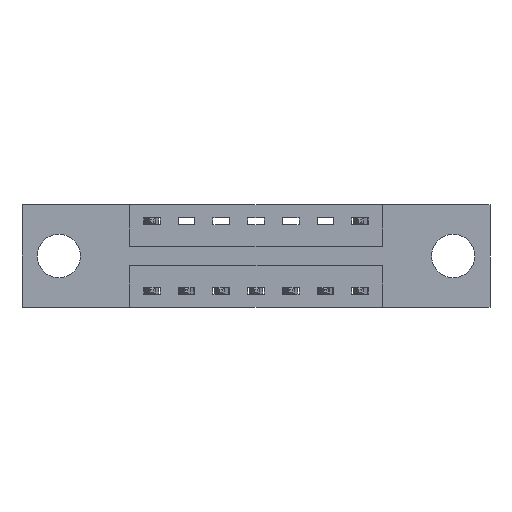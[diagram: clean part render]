
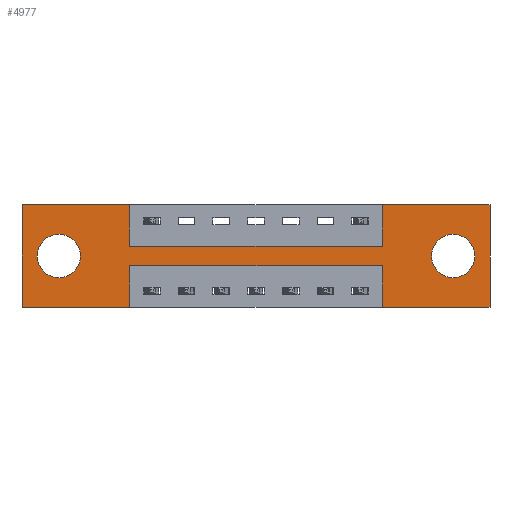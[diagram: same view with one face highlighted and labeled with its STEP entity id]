
A CAD part, front view. The second image highlights one B-rep face of the part: STEP entity #4977.
In plain terms, the highlighted planar face has unit normal (0, -1, 0).
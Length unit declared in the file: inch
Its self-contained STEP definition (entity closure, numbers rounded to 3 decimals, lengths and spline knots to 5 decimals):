
#49 = DIRECTION ( 'NONE',  ( 0., 1., 0. ) ) ;
#117 = CARTESIAN_POINT ( 'NONE',  ( 0.3875, 0., -0.22 ) ) ;
#160 = DIRECTION ( 'NONE',  ( 1., 0., 0. ) ) ;
#253 = FACE_BOUND ( 'NONE', #4351, .T. ) ;
#268 = CARTESIAN_POINT ( 'NONE',  ( 0.3875, 0., 0. ) ) ;
#353 = DIRECTION ( 'NONE',  ( 0., 1., 0. ) ) ;
#394 = LINE ( 'NONE', #3100, #5935 ) ;
#747 = CARTESIAN_POINT ( 'NONE',  ( 1.5525, 0., -0.107 ) ) ;
#950 = VERTEX_POINT ( 'NONE', #7393 ) ;
#989 = CARTESIAN_POINT ( 'NONE',  ( 1.685, 0., -0.37 ) ) ;
#1057 = CARTESIAN_POINT ( 'NONE',  ( 0.1325, 0., -0.263 ) ) ;
#1144 = VECTOR ( 'NONE', #8633, 39.37008 ) ;
#1188 = DIRECTION ( 'NONE',  ( 1., 0., 0. ) ) ;
#1196 = CARTESIAN_POINT ( 'NONE',  ( 1.685, 0., 0. ) ) ;
#1338 = CARTESIAN_POINT ( 'NONE',  ( 1.685, 0., 0. ) ) ;
#1531 = CARTESIAN_POINT ( 'NONE',  ( 1.2975, 0., -0.15 ) ) ;
#1603 = CARTESIAN_POINT ( 'NONE',  ( 0.1325, 0., -0.185 ) ) ;
#1684 = VECTOR ( 'NONE', #6977, 39.37008 ) ;
#1796 = EDGE_CURVE ( 'NONE', #6380, #5802, #6871, .T. ) ;
#1917 = LINE ( 'NONE', #8326, #1684 ) ;
#2292 = EDGE_LOOP ( 'NONE', ( #3022, #3030 ) ) ;
#2313 = DIRECTION ( 'NONE',  ( 0., 0., 1. ) ) ;
#2333 = CIRCLE ( 'NONE', #7362, 0.078 ) ;
#2462 = CARTESIAN_POINT ( 'NONE',  ( 1.2975, 0., 0. ) ) ;
#2491 = CARTESIAN_POINT ( 'NONE',  ( 0.3875, 0., -0.15 ) ) ;
#2604 = LINE ( 'NONE', #8018, #6604 ) ;
#2823 = EDGE_CURVE ( 'NONE', #4081, #3198, #4790, .T. ) ;
#2849 = DIRECTION ( 'NONE',  ( 0., 0., 1. ) ) ;
#2854 = EDGE_CURVE ( 'NONE', #950, #4915, #2604, .T. ) ;
#2866 = CARTESIAN_POINT ( 'NONE',  ( 1.2975, 0., -0.37 ) ) ;
#2938 = EDGE_CURVE ( 'NONE', #8661, #8866, #8307, .T. ) ;
#2955 = ORIENTED_EDGE ( 'NONE', *, *, #4554, .T. ) ;
#2957 = LINE ( 'NONE', #7726, #5098 ) ;
#2965 = ORIENTED_EDGE ( 'NONE', *, *, #5961, .T. ) ;
#3022 = ORIENTED_EDGE ( 'NONE', *, *, #4556, .T. ) ;
#3028 = EDGE_CURVE ( 'NONE', #3198, #8661, #3564, .T. ) ;
#3030 = ORIENTED_EDGE ( 'NONE', *, *, #7304, .T. ) ;
#3062 = ORIENTED_EDGE ( 'NONE', *, *, #4607, .F. ) ;
#3074 = DIRECTION ( 'NONE',  ( 0., 0., -1. ) ) ;
#3100 = CARTESIAN_POINT ( 'NONE',  ( 0.3875, 0., -0.37 ) ) ;
#3119 = ORIENTED_EDGE ( 'NONE', *, *, #4675, .F. ) ;
#3121 = VECTOR ( 'NONE', #2849, 39.37008 ) ;
#3140 = ORIENTED_EDGE ( 'NONE', *, *, #1796, .F. ) ;
#3196 = ORIENTED_EDGE ( 'NONE', *, *, #4365, .F. ) ;
#3198 = VERTEX_POINT ( 'NONE', #1531 ) ;
#3221 = ORIENTED_EDGE ( 'NONE', *, *, #4212, .F. ) ;
#3258 = VERTEX_POINT ( 'NONE', #7922 ) ;
#3302 = ORIENTED_EDGE ( 'NONE', *, *, #2938, .F. ) ;
#3335 = ORIENTED_EDGE ( 'NONE', *, *, #3028, .F. ) ;
#3381 = ORIENTED_EDGE ( 'NONE', *, *, #2823, .F. ) ;
#3429 = VERTEX_POINT ( 'NONE', #989 ) ;
#3437 = ORIENTED_EDGE ( 'NONE', *, *, #3493, .F. ) ;
#3493 = EDGE_CURVE ( 'NONE', #4915, #4081, #5617, .T. ) ;
#3506 = ORIENTED_EDGE ( 'NONE', *, *, #2854, .F. ) ;
#3527 = CARTESIAN_POINT ( 'NONE',  ( 1.2975, 0., 0. ) ) ;
#3564 = LINE ( 'NONE', #3527, #8788 ) ;
#3596 = DIRECTION ( 'NONE',  ( -1., 0., 0. ) ) ;
#3646 = ORIENTED_EDGE ( 'NONE', *, *, #4149, .F. ) ;
#3649 = ORIENTED_EDGE ( 'NONE', *, *, #4467, .F. ) ;
#3862 = CARTESIAN_POINT ( 'NONE',  ( 0.3875, 0., -0.15 ) ) ;
#3903 = DIRECTION ( 'NONE',  ( 0., 1., 0. ) ) ;
#4070 = VERTEX_POINT ( 'NONE', #6737 ) ;
#4081 = VERTEX_POINT ( 'NONE', #2491 ) ;
#4085 = VERTEX_POINT ( 'NONE', #7424 ) ;
#4101 = LINE ( 'NONE', #117, #5712 ) ;
#4149 = EDGE_CURVE ( 'NONE', #4070, #950, #5416, .T. ) ;
#4212 = EDGE_CURVE ( 'NONE', #8866, #3429, #4552, .T. ) ;
#4321 = CIRCLE ( 'NONE', #6446, 0.078 ) ;
#4351 = EDGE_LOOP ( 'NONE', ( #2955, #2965 ) ) ;
#4365 = EDGE_CURVE ( 'NONE', #3429, #6380, #1917, .T. ) ;
#4404 = CARTESIAN_POINT ( 'NONE',  ( 1.5525, 0., -0.185 ) ) ;
#4467 = EDGE_CURVE ( 'NONE', #3258, #4070, #2957, .T. ) ;
#4552 = LINE ( 'NONE', #1196, #8180 ) ;
#4554 = EDGE_CURVE ( 'NONE', #6246, #4085, #4321, .T. ) ;
#4556 = EDGE_CURVE ( 'NONE', #6906, #8626, #2333, .T. ) ;
#4560 = VERTEX_POINT ( 'NONE', #7817 ) ;
#4590 = DIRECTION ( 'NONE',  ( -1., 0., 0. ) ) ;
#4607 = EDGE_CURVE ( 'NONE', #4560, #3258, #394, .T. ) ;
#4675 = EDGE_CURVE ( 'NONE', #5802, #4560, #4101, .T. ) ;
#4745 = DIRECTION ( 'NONE',  ( 0., 0., 1. ) ) ;
#4762 = CARTESIAN_POINT ( 'NONE',  ( 1.5525, 0., -0.185 ) ) ;
#4769 = CARTESIAN_POINT ( 'NONE',  ( 0., 0., 0. ) ) ;
#4770 = CARTESIAN_POINT ( 'NONE',  ( 0.3875, 0., 0. ) ) ;
#4790 = LINE ( 'NONE', #3862, #1144 ) ;
#4915 = VERTEX_POINT ( 'NONE', #4770 ) ;
#4951 = CIRCLE ( 'NONE', #7723, 0.078 ) ;
#4977 = ADVANCED_FACE ( 'NONE', ( #253, #5404, #8958 ), #6554, .T. ) ;
#5098 = VECTOR ( 'NONE', #3596, 39.37008 ) ;
#5221 = CARTESIAN_POINT ( 'NONE',  ( 1.2975, 0., -0.22 ) ) ;
#5228 = DIRECTION ( 'NONE',  ( 0., 0., -1. ) ) ;
#5375 = AXIS2_PLACEMENT_3D ( 'NONE', #5871, #7246, #3074 ) ;
#5404 = FACE_BOUND ( 'NONE', #2292, .T. ) ;
#5416 = LINE ( 'NONE', #8783, #6057 ) ;
#5454 = DIRECTION ( 'NONE',  ( 0., 0., -1. ) ) ;
#5617 = LINE ( 'NONE', #268, #8968 ) ;
#5712 = VECTOR ( 'NONE', #4590, 39.37008 ) ;
#5802 = VERTEX_POINT ( 'NONE', #5221 ) ;
#5871 = CARTESIAN_POINT ( 'NONE',  ( 0., 0., -0.37 ) ) ;
#5903 = DIRECTION ( 'NONE',  ( 0., 0., -1. ) ) ;
#5935 = VECTOR ( 'NONE', #5903, 39.37008 ) ;
#5961 = EDGE_CURVE ( 'NONE', #4085, #6246, #7525, .T. ) ;
#6057 = VECTOR ( 'NONE', #4745, 39.37008 ) ;
#6205 = DIRECTION ( 'NONE',  ( 0., 0., -1. ) ) ;
#6246 = VERTEX_POINT ( 'NONE', #747 ) ;
#6300 = DIRECTION ( 'NONE',  ( 0., 0., 1. ) ) ;
#6380 = VERTEX_POINT ( 'NONE', #8594 ) ;
#6446 = AXIS2_PLACEMENT_3D ( 'NONE', #4404, #49, #5228 ) ;
#6554 = PLANE ( 'NONE',  #5375 ) ;
#6584 = DIRECTION ( 'NONE',  ( 0., 1., 0. ) ) ;
#6604 = VECTOR ( 'NONE', #160, 39.37008 ) ;
#6737 = CARTESIAN_POINT ( 'NONE',  ( 0., 0., -0.37 ) ) ;
#6837 = EDGE_LOOP ( 'NONE', ( #3062, #3119, #3140, #3196, #3221, #3302, #3335, #3381, #3437, #3506, #3646, #3649 ) ) ;
#6871 = LINE ( 'NONE', #2866, #3121 ) ;
#6906 = VERTEX_POINT ( 'NONE', #9102 ) ;
#6977 = DIRECTION ( 'NONE',  ( -1., 0., 0. ) ) ;
#7246 = DIRECTION ( 'NONE',  ( 0., -1., 0. ) ) ;
#7304 = EDGE_CURVE ( 'NONE', #8626, #6906, #4951, .T. ) ;
#7362 = AXIS2_PLACEMENT_3D ( 'NONE', #1603, #6584, #2313 ) ;
#7393 = CARTESIAN_POINT ( 'NONE',  ( 0., 0., 0. ) ) ;
#7424 = CARTESIAN_POINT ( 'NONE',  ( 1.5525, 0., -0.263 ) ) ;
#7525 = CIRCLE ( 'NONE', #7770, 0.078 ) ;
#7723 = AXIS2_PLACEMENT_3D ( 'NONE', #8022, #3903, #8665 ) ;
#7726 = CARTESIAN_POINT ( 'NONE',  ( 0., 0., -0.37 ) ) ;
#7770 = AXIS2_PLACEMENT_3D ( 'NONE', #4762, #353, #5454 ) ;
#7817 = CARTESIAN_POINT ( 'NONE',  ( 0.3875, 0., -0.22 ) ) ;
#7922 = CARTESIAN_POINT ( 'NONE',  ( 0.3875, 0., -0.37 ) ) ;
#8018 = CARTESIAN_POINT ( 'NONE',  ( 0., 0., 0. ) ) ;
#8022 = CARTESIAN_POINT ( 'NONE',  ( 0.1325, 0., -0.185 ) ) ;
#8081 = VECTOR ( 'NONE', #1188, 39.37008 ) ;
#8180 = VECTOR ( 'NONE', #6205, 39.37008 ) ;
#8307 = LINE ( 'NONE', #4769, #8081 ) ;
#8326 = CARTESIAN_POINT ( 'NONE',  ( 0., 0., -0.37 ) ) ;
#8594 = CARTESIAN_POINT ( 'NONE',  ( 1.2975, 0., -0.37 ) ) ;
#8626 = VERTEX_POINT ( 'NONE', #1057 ) ;
#8633 = DIRECTION ( 'NONE',  ( 1., 0., 0. ) ) ;
#8661 = VERTEX_POINT ( 'NONE', #2462 ) ;
#8665 = DIRECTION ( 'NONE',  ( 0., 0., 1. ) ) ;
#8736 = DIRECTION ( 'NONE',  ( 0., 0., -1. ) ) ;
#8783 = CARTESIAN_POINT ( 'NONE',  ( 0., 0., 0. ) ) ;
#8788 = VECTOR ( 'NONE', #6300, 39.37008 ) ;
#8866 = VERTEX_POINT ( 'NONE', #1338 ) ;
#8958 = FACE_OUTER_BOUND ( 'NONE', #6837, .T. ) ;
#8968 = VECTOR ( 'NONE', #8736, 39.37008 ) ;
#9102 = CARTESIAN_POINT ( 'NONE',  ( 0.1325, 0., -0.107 ) ) ;
